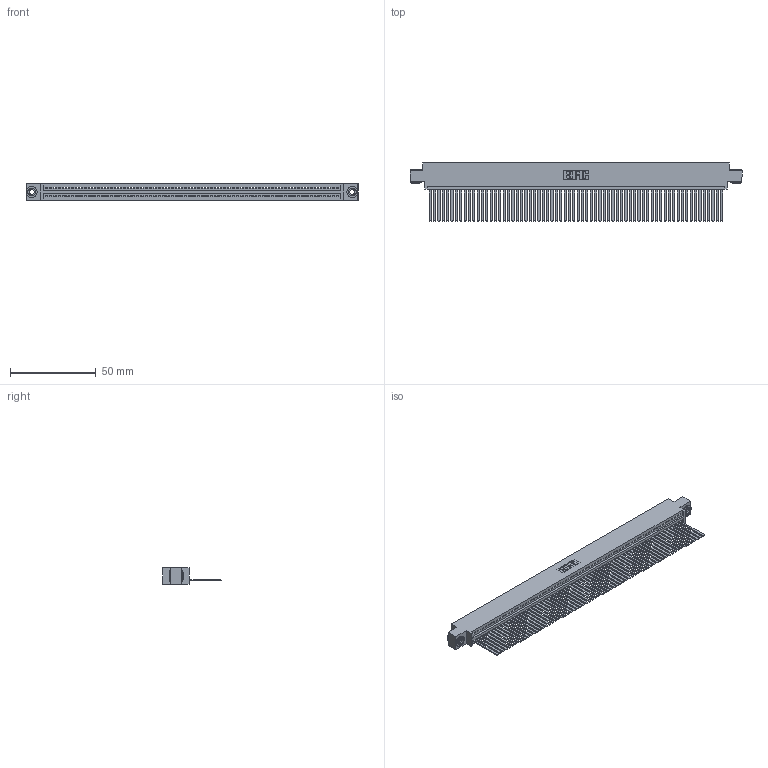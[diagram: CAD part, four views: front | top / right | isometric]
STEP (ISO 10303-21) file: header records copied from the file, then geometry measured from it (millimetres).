
FILE_DESCRIPTION (( 'STEP AP203' ), '1' );
FILE_NAME ('395-068-544-603.STEP', '2018-11-25T18:17:04', ( '' ), ( '' ), 'SwSTEP 2.0', 'SolidWorks 2016', '' );
FILE_SCHEMA (( 'CONFIG_CONTROL_DESIGN' ));
Length unit declared in the file: inch
Products named in the file (4): 345-250-002_345-250-002-102; 345-292-001_345-293-144; 345 Part_0.170 Offset - 0.156 Dia-TH; 395-068-544-603
Assembly tree (71 placements, depth 2):
  395-068-544-603
    345 Part_0.170 Offset - 0.156 Dia-TH
    345-292-001_345-293-144  x68
    345-250-002_345-250-002-102  x2
Bounding box: 193.93 x 33.96 x 9.4 mm (x, y, z)
Volume: 19326.1 mm3; surface area: 28741.3 mm2
Topology: 71 solids, 71 shells, 3704 faces, 11173 edges, 7354 vertices
Faces by surface type: plane 2542, cylinder 1154, cone 8
Entity records: 48276 total; most frequent: CARTESIAN_POINT 8339, ORIENTED_EDGE 8334, DIRECTION 7273, EDGE_CURVE 4167, VECTOR 3743, LINE 3743, VERTEX_POINT 2774, AXIS2_PLACEMENT_3D 1765
